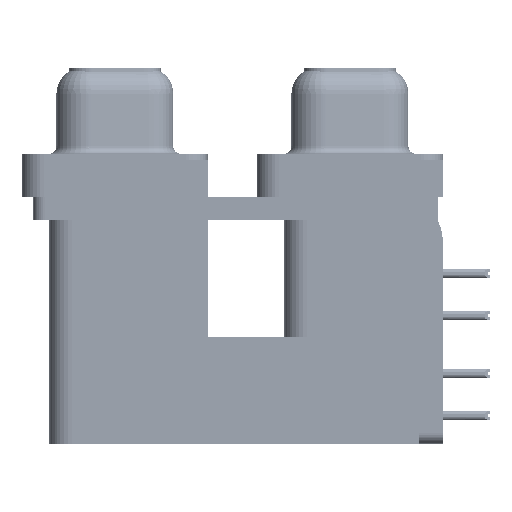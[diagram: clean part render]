
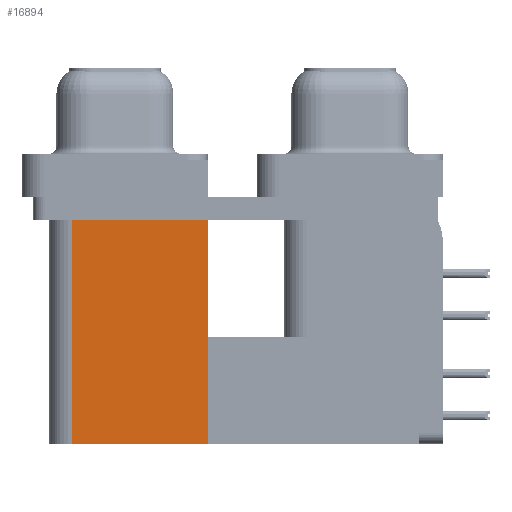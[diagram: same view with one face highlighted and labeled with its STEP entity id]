
A CAD part, left-side view. The second image highlights one B-rep face of the part: STEP entity #16894.
In plain terms, the highlighted planar face has unit normal (-1, 0, 0).
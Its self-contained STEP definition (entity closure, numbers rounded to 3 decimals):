
#1180 = VECTOR ( 'NONE', #70181, 1000. ) ;
#1349 = PLANE ( 'NONE',  #16861 ) ;
#2320 = EDGE_LOOP ( 'NONE', ( #27999, #28743, #60415, #69362 ) ) ;
#2641 = VECTOR ( 'NONE', #37296, 1000. ) ;
#6173 = VECTOR ( 'NONE', #26055, 1000. ) ;
#6844 = CARTESIAN_POINT ( 'NONE',  ( 3.79, 9.6, -19.2 ) ) ;
#8646 = VERTEX_POINT ( 'NONE', #6844 ) ;
#9265 = LINE ( 'NONE', #53700, #2641 ) ;
#12106 = EDGE_CURVE ( 'NONE', #8646, #71674, #69421, .T. ) ;
#12204 = VERTEX_POINT ( 'NONE', #44981 ) ;
#12640 = DIRECTION ( 'NONE',  ( 0., 0., -1. ) ) ;
#14430 = CARTESIAN_POINT ( 'NONE',  ( 3.79, 9.6, -19.2 ) ) ;
#16861 = AXIS2_PLACEMENT_3D ( 'NONE', #38881, #50181, #12640 ) ;
#16894 = ADVANCED_FACE ( 'NONE', ( #45087 ), #1349, .F. ) ;
#18451 = CARTESIAN_POINT ( 'NONE',  ( 3.79, 18.8, -19.2 ) ) ;
#23924 = VERTEX_POINT ( 'NONE', #18451 ) ;
#25335 = CARTESIAN_POINT ( 'NONE',  ( 3.79, 9.6, -19.2 ) ) ;
#26055 = DIRECTION ( 'NONE',  ( 0., 0., 1. ) ) ;
#26763 = LINE ( 'NONE', #14430, #57968 ) ;
#26966 = EDGE_CURVE ( 'NONE', #8646, #23924, #26763, .T. ) ;
#27999 = ORIENTED_EDGE ( 'NONE', *, *, #33667, .T. ) ;
#28743 = ORIENTED_EDGE ( 'NONE', *, *, #29699, .F. ) ;
#29699 = EDGE_CURVE ( 'NONE', #23924, #12204, #41811, .T. ) ;
#33667 = EDGE_CURVE ( 'NONE', #71674, #12204, #9265, .T. ) ;
#37296 = DIRECTION ( 'NONE',  ( 0., 1., 0. ) ) ;
#37743 = CARTESIAN_POINT ( 'NONE',  ( 3.79, 18.8, -19.2 ) ) ;
#38881 = CARTESIAN_POINT ( 'NONE',  ( 3.79, 9.6, -19.2 ) ) ;
#41811 = LINE ( 'NONE', #37743, #1180 ) ;
#42291 = CARTESIAN_POINT ( 'NONE',  ( 3.79, 9.6, -2.5 ) ) ;
#44981 = CARTESIAN_POINT ( 'NONE',  ( 3.79, 18.8, -2.5 ) ) ;
#45087 = FACE_OUTER_BOUND ( 'NONE', #2320, .T. ) ;
#50181 = DIRECTION ( 'NONE',  ( 1., 0., 0. ) ) ;
#53700 = CARTESIAN_POINT ( 'NONE',  ( 3.79, 9.6, -2.5 ) ) ;
#57968 = VECTOR ( 'NONE', #69771, 1000. ) ;
#60415 = ORIENTED_EDGE ( 'NONE', *, *, #26966, .F. ) ;
#69362 = ORIENTED_EDGE ( 'NONE', *, *, #12106, .T. ) ;
#69421 = LINE ( 'NONE', #25335, #6173 ) ;
#69771 = DIRECTION ( 'NONE',  ( 0., 1., 0. ) ) ;
#70181 = DIRECTION ( 'NONE',  ( 0., 0., 1. ) ) ;
#71674 = VERTEX_POINT ( 'NONE', #42291 ) ;
